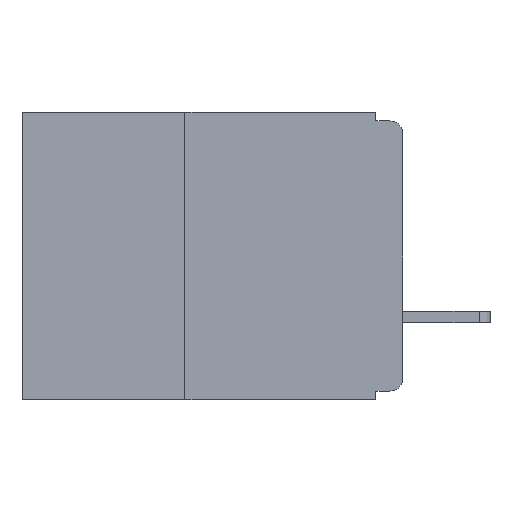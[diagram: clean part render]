
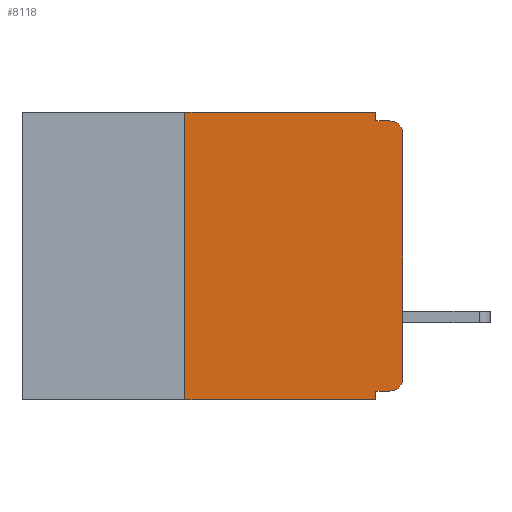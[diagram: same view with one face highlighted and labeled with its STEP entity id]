
A CAD part, left-side view. The second image highlights one B-rep face of the part: STEP entity #8118.
In plain terms, the highlighted planar face has unit normal (-1, 0, 0).
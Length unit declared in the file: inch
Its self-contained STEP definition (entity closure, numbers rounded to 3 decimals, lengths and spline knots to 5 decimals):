
#35 = CARTESIAN_POINT ( 'NONE',  ( 0., 0.031, -0.01 ) ) ;
#478 = AXIS2_PLACEMENT_3D ( 'NONE', #14743, #21810, #11392 ) ;
#798 = LINE ( 'NONE', #17063, #1339 ) ;
#810 = VERTEX_POINT ( 'NONE', #7999 ) ;
#846 = DIRECTION ( 'NONE',  ( 0., -1., 0. ) ) ;
#1339 = VECTOR ( 'NONE', #4835, 39.37008 ) ;
#1432 = DIRECTION ( 'NONE',  ( 0., -1., 0. ) ) ;
#1499 = CARTESIAN_POINT ( 'NONE',  ( 0., 0.437, 0. ) ) ;
#2221 = AXIS2_PLACEMENT_3D ( 'NONE', #6846, #19068, #8582 ) ;
#2500 = ORIENTED_EDGE ( 'NONE', *, *, #21233, .T. ) ;
#2808 = CARTESIAN_POINT ( 'NONE',  ( 0., 0.015, -0.01 ) ) ;
#3022 = VECTOR ( 'NONE', #8364, 39.37008 ) ;
#3032 = ORIENTED_EDGE ( 'NONE', *, *, #4310, .F. ) ;
#3344 = EDGE_CURVE ( 'NONE', #3962, #15222, #21277, .T. ) ;
#3583 = LINE ( 'NONE', #6630, #3022 ) ;
#3962 = VERTEX_POINT ( 'NONE', #6440 ) ;
#4106 = ORIENTED_EDGE ( 'NONE', *, *, #15783, .F. ) ;
#4310 = EDGE_CURVE ( 'NONE', #15780, #810, #19598, .T. ) ;
#4415 = VERTEX_POINT ( 'NONE', #35 ) ;
#4835 = DIRECTION ( 'NONE',  ( 0., 0., -1. ) ) ;
#4905 = CARTESIAN_POINT ( 'NONE',  ( 0., 0.25, 0. ) ) ;
#5353 = CIRCLE ( 'NONE', #2221, 0.015 ) ;
#5848 = LINE ( 'NONE', #12098, #9979 ) ;
#6379 = CARTESIAN_POINT ( 'NONE',  ( 0., 0., -0.305 ) ) ;
#6440 = CARTESIAN_POINT ( 'NONE',  ( 0., 0.015, -0.32 ) ) ;
#6630 = CARTESIAN_POINT ( 'NONE',  ( 0., 0.25, -0.33 ) ) ;
#6846 = CARTESIAN_POINT ( 'NONE',  ( 0., 0.015, -0.025 ) ) ;
#7078 = ORIENTED_EDGE ( 'NONE', *, *, #9563, .F. ) ;
#7579 = VECTOR ( 'NONE', #846, 39.37008 ) ;
#7603 = VECTOR ( 'NONE', #22315, 39.37008 ) ;
#7999 = CARTESIAN_POINT ( 'NONE',  ( 0., 0.031, 0. ) ) ;
#8118 = ADVANCED_FACE ( 'NONE', ( #22151 ), #9604, .F. ) ;
#8364 = DIRECTION ( 'NONE',  ( 0., 0., 1. ) ) ;
#8410 = DIRECTION ( 'NONE',  ( 0., 0., -1. ) ) ;
#8582 = DIRECTION ( 'NONE',  ( 0., 0., -1. ) ) ;
#8586 = VERTEX_POINT ( 'NONE', #12742 ) ;
#9261 = ORIENTED_EDGE ( 'NONE', *, *, #3344, .T. ) ;
#9563 = EDGE_CURVE ( 'NONE', #4415, #12105, #5848, .T. ) ;
#9604 = PLANE ( 'NONE',  #478 ) ;
#9888 = EDGE_LOOP ( 'NONE', ( #10632, #2500, #7078, #11736, #3032, #12290, #17486, #4106, #13395, #9261 ) ) ;
#9979 = VECTOR ( 'NONE', #15621, 39.37008 ) ;
#10103 = CARTESIAN_POINT ( 'NONE',  ( 0., 0.031, -0.33 ) ) ;
#10186 = VECTOR ( 'NONE', #14193, 39.37008 ) ;
#10548 = VERTEX_POINT ( 'NONE', #19015 ) ;
#10632 = ORIENTED_EDGE ( 'NONE', *, *, #14860, .T. ) ;
#11197 = CARTESIAN_POINT ( 'NONE',  ( 0., 0.437, -0.33 ) ) ;
#11392 = DIRECTION ( 'NONE',  ( 0., 0., -1. ) ) ;
#11736 = ORIENTED_EDGE ( 'NONE', *, *, #20004, .F. ) ;
#12098 = CARTESIAN_POINT ( 'NONE',  ( 0., 0., -0.01 ) ) ;
#12105 = VERTEX_POINT ( 'NONE', #2808 ) ;
#12290 = ORIENTED_EDGE ( 'NONE', *, *, #17681, .F. ) ;
#12742 = CARTESIAN_POINT ( 'NONE',  ( 0., 0.031, -0.33 ) ) ;
#13042 = CARTESIAN_POINT ( 'NONE',  ( 0., 0., -0.025 ) ) ;
#13395 = ORIENTED_EDGE ( 'NONE', *, *, #17684, .F. ) ;
#14125 = CARTESIAN_POINT ( 'NONE',  ( 0., 0., 0. ) ) ;
#14132 = DIRECTION ( 'NONE',  ( 0., 0., -1. ) ) ;
#14148 = DIRECTION ( 'NONE',  ( -1., 0., 0. ) ) ;
#14193 = DIRECTION ( 'NONE',  ( 0., 0., 1. ) ) ;
#14245 = CARTESIAN_POINT ( 'NONE',  ( 0., 0.015, -0.305 ) ) ;
#14409 = VECTOR ( 'NONE', #1432, 39.37008 ) ;
#14743 = CARTESIAN_POINT ( 'NONE',  ( 0., 0.437, 0. ) ) ;
#14781 = VECTOR ( 'NONE', #8410, 39.37008 ) ;
#14860 = EDGE_CURVE ( 'NONE', #15222, #15051, #19465, .T. ) ;
#15051 = VERTEX_POINT ( 'NONE', #13042 ) ;
#15222 = VERTEX_POINT ( 'NONE', #6379 ) ;
#15229 = AXIS2_PLACEMENT_3D ( 'NONE', #14245, #14148, #14132 ) ;
#15358 = LINE ( 'NONE', #10103, #14781 ) ;
#15621 = DIRECTION ( 'NONE',  ( 0., -1., 0. ) ) ;
#15780 = VERTEX_POINT ( 'NONE', #4905 ) ;
#15783 = EDGE_CURVE ( 'NONE', #22395, #8586, #15358, .T. ) ;
#17063 = CARTESIAN_POINT ( 'NONE',  ( 0., 0.031, 0. ) ) ;
#17486 = ORIENTED_EDGE ( 'NONE', *, *, #18117, .T. ) ;
#17681 = EDGE_CURVE ( 'NONE', #10548, #15780, #3583, .T. ) ;
#17684 = EDGE_CURVE ( 'NONE', #3962, #22395, #22082, .T. ) ;
#18117 = EDGE_CURVE ( 'NONE', #10548, #8586, #21505, .T. ) ;
#19015 = CARTESIAN_POINT ( 'NONE',  ( 0., 0.25, -0.33 ) ) ;
#19068 = DIRECTION ( 'NONE',  ( -1., 0., 0. ) ) ;
#19465 = LINE ( 'NONE', #14125, #10186 ) ;
#19598 = LINE ( 'NONE', #1499, #14409 ) ;
#20004 = EDGE_CURVE ( 'NONE', #810, #4415, #798, .T. ) ;
#20600 = CARTESIAN_POINT ( 'NONE',  ( 0., 0., -0.32 ) ) ;
#21233 = EDGE_CURVE ( 'NONE', #15051, #12105, #5353, .T. ) ;
#21277 = CIRCLE ( 'NONE', #15229, 0.015 ) ;
#21505 = LINE ( 'NONE', #11197, #7579 ) ;
#21810 = DIRECTION ( 'NONE',  ( 1., 0., 0. ) ) ;
#21877 = CARTESIAN_POINT ( 'NONE',  ( 0., 0.031, -0.32 ) ) ;
#22082 = LINE ( 'NONE', #20600, #7603 ) ;
#22151 = FACE_OUTER_BOUND ( 'NONE', #9888, .T. ) ;
#22315 = DIRECTION ( 'NONE',  ( 0., 1., 0. ) ) ;
#22395 = VERTEX_POINT ( 'NONE', #21877 ) ;
